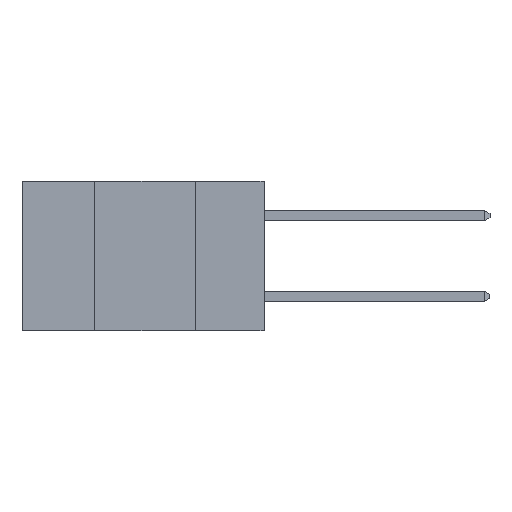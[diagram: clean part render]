
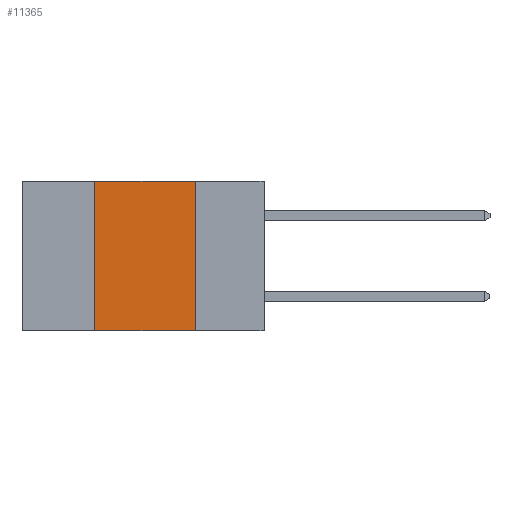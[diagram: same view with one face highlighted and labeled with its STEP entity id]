
A CAD part, left-side view. The second image highlights one B-rep face of the part: STEP entity #11365.
In plain terms, the highlighted planar face has unit normal (-1, 0, 0).
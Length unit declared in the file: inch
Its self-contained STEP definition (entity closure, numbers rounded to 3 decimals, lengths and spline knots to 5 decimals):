
#1401 = ORIENTED_EDGE ( 'NONE', *, *, #23588, .F. ) ;
#2261 = CARTESIAN_POINT ( 'NONE',  ( 0., 0.42, -0.37 ) ) ;
#2411 = VECTOR ( 'NONE', #11681, 39.37008 ) ;
#2862 = DIRECTION ( 'NONE',  ( 0., -1., 0. ) ) ;
#4009 = AXIS2_PLACEMENT_3D ( 'NONE', #10687, #29569, #15480 ) ;
#4363 = VERTEX_POINT ( 'NONE', #29346 ) ;
#4461 = DIRECTION ( 'NONE',  ( 0., -1., 0. ) ) ;
#4608 = CARTESIAN_POINT ( 'NONE',  ( 0., 0.17, 0. ) ) ;
#4864 = CARTESIAN_POINT ( 'NONE',  ( 0., 0.17, -0.37 ) ) ;
#4898 = CARTESIAN_POINT ( 'NONE',  ( 0., 0.42, 0. ) ) ;
#7148 = VECTOR ( 'NONE', #28216, 39.37008 ) ;
#8692 = EDGE_CURVE ( 'NONE', #4363, #30135, #27642, .T. ) ;
#8922 = VECTOR ( 'NONE', #4461, 39.37008 ) ;
#10687 = CARTESIAN_POINT ( 'NONE',  ( 0., 0.6, 0. ) ) ;
#11365 = ADVANCED_FACE ( 'NONE', ( #12368 ), #24899, .F. ) ;
#11530 = CARTESIAN_POINT ( 'NONE',  ( 0., 0.6, 0. ) ) ;
#11681 = DIRECTION ( 'NONE',  ( 0., 0., -1. ) ) ;
#11864 = EDGE_CURVE ( 'NONE', #24860, #30135, #17199, .T. ) ;
#12337 = VECTOR ( 'NONE', #2862, 39.37008 ) ;
#12368 = FACE_OUTER_BOUND ( 'NONE', #13694, .T. ) ;
#12968 = EDGE_CURVE ( 'NONE', #24915, #4363, #15231, .T. ) ;
#13694 = EDGE_LOOP ( 'NONE', ( #23283, #17401, #1401, #15048 ) ) ;
#15048 = ORIENTED_EDGE ( 'NONE', *, *, #11864, .T. ) ;
#15231 = LINE ( 'NONE', #11530, #8922 ) ;
#15480 = DIRECTION ( 'NONE',  ( 0., 0., -1. ) ) ;
#17199 = LINE ( 'NONE', #19517, #12337 ) ;
#17401 = ORIENTED_EDGE ( 'NONE', *, *, #12968, .F. ) ;
#19517 = CARTESIAN_POINT ( 'NONE',  ( 0., 0.6, -0.37 ) ) ;
#23283 = ORIENTED_EDGE ( 'NONE', *, *, #8692, .F. ) ;
#23588 = EDGE_CURVE ( 'NONE', #24860, #24915, #26026, .T. ) ;
#24860 = VERTEX_POINT ( 'NONE', #2261 ) ;
#24899 = PLANE ( 'NONE',  #4009 ) ;
#24915 = VERTEX_POINT ( 'NONE', #4898 ) ;
#25878 = CARTESIAN_POINT ( 'NONE',  ( 0., 0.42, 0. ) ) ;
#26026 = LINE ( 'NONE', #25878, #7148 ) ;
#27642 = LINE ( 'NONE', #4608, #2411 ) ;
#28216 = DIRECTION ( 'NONE',  ( 0., 0., 1. ) ) ;
#29346 = CARTESIAN_POINT ( 'NONE',  ( 0., 0.17, 0. ) ) ;
#29569 = DIRECTION ( 'NONE',  ( 1., 0., 0. ) ) ;
#30135 = VERTEX_POINT ( 'NONE', #4864 ) ;
